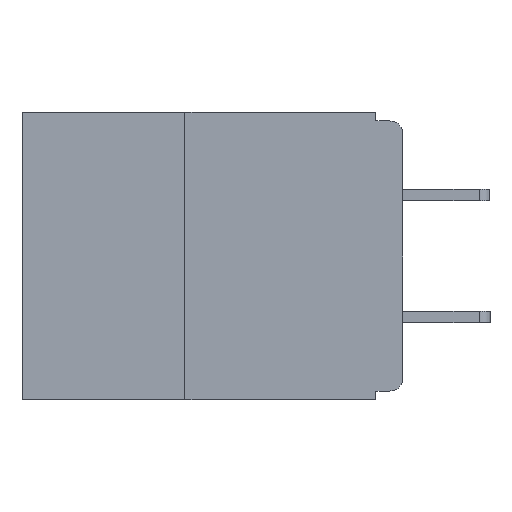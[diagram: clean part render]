
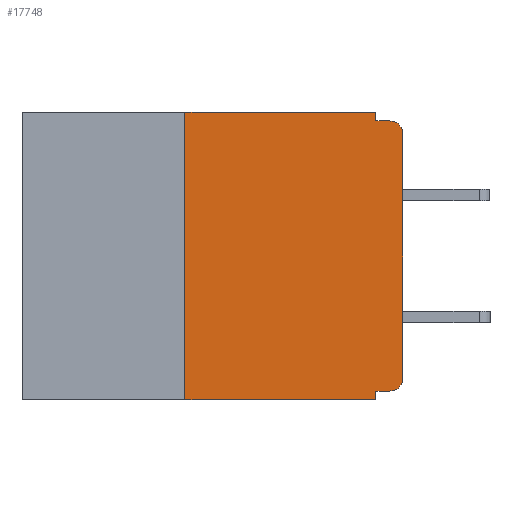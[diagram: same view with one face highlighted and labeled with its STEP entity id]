
A CAD part, left-side view. The second image highlights one B-rep face of the part: STEP entity #17748.
In plain terms, the highlighted planar face has unit normal (-1, 0, 0).
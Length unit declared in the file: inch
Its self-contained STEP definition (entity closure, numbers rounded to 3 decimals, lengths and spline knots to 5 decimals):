
#11 = CARTESIAN_POINT ( 'NONE',  ( 0., 0.031, -0.33 ) ) ;
#43 = VECTOR ( 'NONE', #4751, 39.37008 ) ;
#233 = CARTESIAN_POINT ( 'NONE',  ( 0., 0., -0.305 ) ) ;
#332 = EDGE_LOOP ( 'NONE', ( #13389, #6018, #10998, #13206, #6950, #15442, #4933, #5355, #10570, #3810 ) ) ;
#380 = LINE ( 'NONE', #5516, #8046 ) ;
#532 = LINE ( 'NONE', #5084, #11540 ) ;
#1239 = EDGE_CURVE ( 'NONE', #1286, #2647, #380, .T. ) ;
#1286 = VERTEX_POINT ( 'NONE', #1707 ) ;
#1593 = CARTESIAN_POINT ( 'NONE',  ( 0., 0.031, -0.33 ) ) ;
#1707 = CARTESIAN_POINT ( 'NONE',  ( 0., 0.015, -0.32 ) ) ;
#2068 = AXIS2_PLACEMENT_3D ( 'NONE', #13152, #4583, #14567 ) ;
#2150 = CIRCLE ( 'NONE', #2068, 0.015 ) ;
#2647 = VERTEX_POINT ( 'NONE', #4093 ) ;
#3368 = CARTESIAN_POINT ( 'NONE',  ( 0., 0.25, -0.33 ) ) ;
#3810 = ORIENTED_EDGE ( 'NONE', *, *, #17025, .T. ) ;
#4093 = CARTESIAN_POINT ( 'NONE',  ( 0., 0.031, -0.32 ) ) ;
#4274 = VERTEX_POINT ( 'NONE', #6519 ) ;
#4303 = CARTESIAN_POINT ( 'NONE',  ( 0., 0.25, -0.33 ) ) ;
#4583 = DIRECTION ( 'NONE',  ( -1., 0., 0. ) ) ;
#4751 = DIRECTION ( 'NONE',  ( 0., -1., 0. ) ) ;
#4796 = LINE ( 'NONE', #11921, #43 ) ;
#4818 = DIRECTION ( 'NONE',  ( 0., 0., 1. ) ) ;
#4933 = ORIENTED_EDGE ( 'NONE', *, *, #9367, .T. ) ;
#5053 = CIRCLE ( 'NONE', #15218, 0.015 ) ;
#5084 = CARTESIAN_POINT ( 'NONE',  ( 0., 0., -0.01 ) ) ;
#5104 = VECTOR ( 'NONE', #7493, 39.37008 ) ;
#5146 = DIRECTION ( 'NONE',  ( 0., -1., 0. ) ) ;
#5355 = ORIENTED_EDGE ( 'NONE', *, *, #16893, .F. ) ;
#5481 = DIRECTION ( 'NONE',  ( 0., 1., 0. ) ) ;
#5516 = CARTESIAN_POINT ( 'NONE',  ( 0., 0., -0.32 ) ) ;
#5529 = LINE ( 'NONE', #6045, #5104 ) ;
#5663 = VERTEX_POINT ( 'NONE', #4303 ) ;
#5859 = CARTESIAN_POINT ( 'NONE',  ( 0., 0., 0. ) ) ;
#6018 = ORIENTED_EDGE ( 'NONE', *, *, #17416, .T. ) ;
#6045 = CARTESIAN_POINT ( 'NONE',  ( 0., 0.031, 0. ) ) ;
#6231 = CARTESIAN_POINT ( 'NONE',  ( 0., 0.015, -0.305 ) ) ;
#6496 = AXIS2_PLACEMENT_3D ( 'NONE', #16737, #18150, #9685 ) ;
#6519 = CARTESIAN_POINT ( 'NONE',  ( 0., 0.031, -0.01 ) ) ;
#6554 = VECTOR ( 'NONE', #9087, 39.37008 ) ;
#6851 = LINE ( 'NONE', #1593, #10439 ) ;
#6950 = ORIENTED_EDGE ( 'NONE', *, *, #10523, .F. ) ;
#7493 = DIRECTION ( 'NONE',  ( 0., 0., -1. ) ) ;
#7530 = VERTEX_POINT ( 'NONE', #11 ) ;
#7688 = DIRECTION ( 'NONE',  ( 0., 0., -1. ) ) ;
#8046 = VECTOR ( 'NONE', #5481, 39.37008 ) ;
#8373 = VERTEX_POINT ( 'NONE', #9157 ) ;
#8777 = DIRECTION ( 'NONE',  ( 0., 0., -1. ) ) ;
#8883 = EDGE_CURVE ( 'NONE', #4274, #16106, #532, .T. ) ;
#9087 = DIRECTION ( 'NONE',  ( 0., -1., 0. ) ) ;
#9157 = CARTESIAN_POINT ( 'NONE',  ( 0., 0.25, 0. ) ) ;
#9367 = EDGE_CURVE ( 'NONE', #5663, #7530, #4796, .T. ) ;
#9685 = DIRECTION ( 'NONE',  ( 0., 0., -1. ) ) ;
#9930 = VECTOR ( 'NONE', #4818, 39.37008 ) ;
#10439 = VECTOR ( 'NONE', #8777, 39.37008 ) ;
#10523 = EDGE_CURVE ( 'NONE', #8373, #12609, #13685, .T. ) ;
#10570 = ORIENTED_EDGE ( 'NONE', *, *, #1239, .F. ) ;
#10998 = ORIENTED_EDGE ( 'NONE', *, *, #8883, .F. ) ;
#11082 = CARTESIAN_POINT ( 'NONE',  ( 0., 0., -0.025 ) ) ;
#11336 = CARTESIAN_POINT ( 'NONE',  ( 0., 0.015, -0.01 ) ) ;
#11520 = DIRECTION ( 'NONE',  ( 0., 0., 1. ) ) ;
#11540 = VECTOR ( 'NONE', #5146, 39.37008 ) ;
#11711 = EDGE_CURVE ( 'NONE', #5663, #8373, #13234, .T. ) ;
#11921 = CARTESIAN_POINT ( 'NONE',  ( 0., 0.437, -0.33 ) ) ;
#12609 = VERTEX_POINT ( 'NONE', #16761 ) ;
#12922 = VERTEX_POINT ( 'NONE', #233 ) ;
#13152 = CARTESIAN_POINT ( 'NONE',  ( 0., 0.015, -0.025 ) ) ;
#13206 = ORIENTED_EDGE ( 'NONE', *, *, #15031, .F. ) ;
#13234 = LINE ( 'NONE', #3368, #9930 ) ;
#13389 = ORIENTED_EDGE ( 'NONE', *, *, #16231, .T. ) ;
#13685 = LINE ( 'NONE', #17576, #6554 ) ;
#14399 = FACE_OUTER_BOUND ( 'NONE', #332, .T. ) ;
#14567 = DIRECTION ( 'NONE',  ( 0., 0., -1. ) ) ;
#15031 = EDGE_CURVE ( 'NONE', #12609, #4274, #5529, .T. ) ;
#15218 = AXIS2_PLACEMENT_3D ( 'NONE', #6231, #16220, #7688 ) ;
#15316 = PLANE ( 'NONE',  #6496 ) ;
#15442 = ORIENTED_EDGE ( 'NONE', *, *, #11711, .F. ) ;
#16106 = VERTEX_POINT ( 'NONE', #11336 ) ;
#16220 = DIRECTION ( 'NONE',  ( -1., 0., 0. ) ) ;
#16231 = EDGE_CURVE ( 'NONE', #12922, #16615, #18206, .T. ) ;
#16615 = VERTEX_POINT ( 'NONE', #11082 ) ;
#16737 = CARTESIAN_POINT ( 'NONE',  ( 0., 0.437, 0. ) ) ;
#16761 = CARTESIAN_POINT ( 'NONE',  ( 0., 0.031, 0. ) ) ;
#16893 = EDGE_CURVE ( 'NONE', #2647, #7530, #6851, .T. ) ;
#17025 = EDGE_CURVE ( 'NONE', #1286, #12922, #5053, .T. ) ;
#17416 = EDGE_CURVE ( 'NONE', #16615, #16106, #2150, .T. ) ;
#17576 = CARTESIAN_POINT ( 'NONE',  ( 0., 0.437, 0. ) ) ;
#17748 = ADVANCED_FACE ( 'NONE', ( #14399 ), #15316, .F. ) ;
#17785 = VECTOR ( 'NONE', #11520, 39.37008 ) ;
#18150 = DIRECTION ( 'NONE',  ( 1., 0., 0. ) ) ;
#18206 = LINE ( 'NONE', #5859, #17785 ) ;
